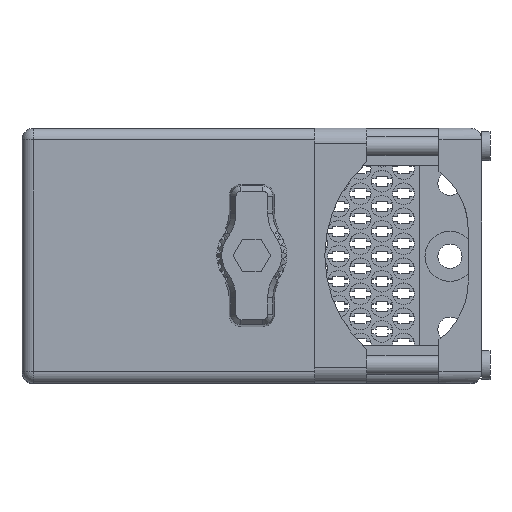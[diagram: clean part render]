
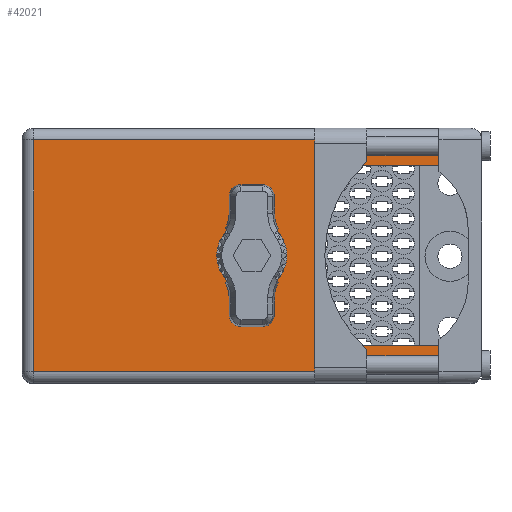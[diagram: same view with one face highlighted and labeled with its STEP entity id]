
A CAD part, top view. The second image highlights one B-rep face of the part: STEP entity #42021.
In plain terms, the highlighted face is planar.
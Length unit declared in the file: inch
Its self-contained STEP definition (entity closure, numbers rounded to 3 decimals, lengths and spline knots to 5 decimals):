
#489 = CARTESIAN_POINT ( 'NONE',  ( 0.4075, 1.93, -0.54 ) ) ;
#1414 = ORIENTED_EDGE ( 'NONE', *, *, #18481, .F. ) ;
#3510 = LINE ( 'NONE', #55622, #70464 ) ;
#4238 = FACE_OUTER_BOUND ( 'NONE', #34804, .T. ) ;
#4299 = VERTEX_POINT ( 'NONE', #4858 ) ;
#4858 = CARTESIAN_POINT ( 'NONE',  ( 1.1215, 1.93, -0.54 ) ) ;
#5364 = DIRECTION ( 'NONE',  ( 0., 0., 1. ) ) ;
#6829 = DIRECTION ( 'NONE',  ( 1., 0., 0. ) ) ;
#6981 = CARTESIAN_POINT ( 'NONE',  ( 1.1215, 1.93, -0.765 ) ) ;
#7824 = DIRECTION ( 'NONE',  ( 0., 1., 0. ) ) ;
#9221 = LINE ( 'NONE', #51453, #51146 ) ;
#11027 = ORIENTED_EDGE ( 'NONE', *, *, #24047, .F. ) ;
#11509 = ORIENTED_EDGE ( 'NONE', *, *, #74046, .F. ) ;
#11756 = DIRECTION ( 'NONE',  ( 0., 0., 1. ) ) ;
#12356 = ORIENTED_EDGE ( 'NONE', *, *, #43190, .T. ) ;
#15482 = CARTESIAN_POINT ( 'NONE',  ( 1.1215, 1.93, -0.695 ) ) ;
#15818 = VERTEX_POINT ( 'NONE', #64501 ) ;
#15840 = DIRECTION ( 'NONE',  ( 0., 0., 1. ) ) ;
#16463 = CARTESIAN_POINT ( 'NONE',  ( -1.3075, 1.93, -0.765 ) ) ;
#17051 = VECTOR ( 'NONE', #6829, 39.37008 ) ;
#18307 = DIRECTION ( 'NONE',  ( -1., 0., 0. ) ) ;
#18397 = CARTESIAN_POINT ( 'NONE',  ( 1.1215, 1.93, -0.765 ) ) ;
#18452 = VERTEX_POINT ( 'NONE', #19703 ) ;
#18481 = EDGE_CURVE ( 'NONE', #60884, #58365, #86616, .T. ) ;
#19607 = VERTEX_POINT ( 'NONE', #54149 ) ;
#19703 = CARTESIAN_POINT ( 'NONE',  ( 1.1215, 1.93, 0.54 ) ) ;
#24047 = EDGE_CURVE ( 'NONE', #58365, #60884, #51631, .T. ) ;
#24074 = VERTEX_POINT ( 'NONE', #76144 ) ;
#25149 = DIRECTION ( 'NONE',  ( 1., 0., 0. ) ) ;
#25889 = VERTEX_POINT ( 'NONE', #37792 ) ;
#26340 = CARTESIAN_POINT ( 'NONE',  ( 1.1215, 1.93, 0.54 ) ) ;
#26749 = VERTEX_POINT ( 'NONE', #50047 ) ;
#28099 = VERTEX_POINT ( 'NONE', #15482 ) ;
#31856 = EDGE_CURVE ( 'NONE', #25889, #26749, #66881, .T. ) ;
#32583 = ORIENTED_EDGE ( 'NONE', *, *, #47386, .T. ) ;
#33002 = LINE ( 'NONE', #18397, #38907 ) ;
#33477 = DIRECTION ( 'NONE',  ( -1., 0., 0. ) ) ;
#34354 = EDGE_CURVE ( 'NONE', #19607, #15818, #55673, .T. ) ;
#34804 = EDGE_LOOP ( 'NONE', ( #63378, #39633, #59728, #93427, #61352, #12356, #11509, #32583 ) ) ;
#37792 = CARTESIAN_POINT ( 'NONE',  ( 0.4075, 1.93, 0.54 ) ) ;
#38254 = CARTESIAN_POINT ( 'NONE',  ( 0., 1.93, 0. ) ) ;
#38815 = VECTOR ( 'NONE', #61947, 39.37008 ) ;
#38907 = VECTOR ( 'NONE', #11756, 39.37008 ) ;
#39633 = ORIENTED_EDGE ( 'NONE', *, *, #98437, .T. ) ;
#39798 = CARTESIAN_POINT ( 'NONE',  ( 0., 1.93, 0.17 ) ) ;
#40092 = AXIS2_PLACEMENT_3D ( 'NONE', #38254, #7824, #15840 ) ;
#42021 = ADVANCED_FACE ( 'NONE', ( #4238, #61637 ), #95406, .T. ) ;
#43190 = EDGE_CURVE ( 'NONE', #26749, #4299, #98501, .T. ) ;
#43706 = CARTESIAN_POINT ( 'NONE',  ( 0., 1.93, -0.17 ) ) ;
#47386 = EDGE_CURVE ( 'NONE', #28099, #19607, #9221, .T. ) ;
#49927 = DIRECTION ( 'NONE',  ( 0., 1., 0. ) ) ;
#50047 = CARTESIAN_POINT ( 'NONE',  ( 0.4075, 1.93, -0.54 ) ) ;
#51146 = VECTOR ( 'NONE', #59412, 39.37008 ) ;
#51198 = DIRECTION ( 'NONE',  ( 0., 1., 0. ) ) ;
#51453 = CARTESIAN_POINT ( 'NONE',  ( -1.3775, 1.93, -0.695 ) ) ;
#51631 = CIRCLE ( 'NONE', #40092, 0.17 ) ;
#52237 = EDGE_CURVE ( 'NONE', #18452, #25889, #86073, .T. ) ;
#53761 = LINE ( 'NONE', #6981, #69246 ) ;
#53992 = DIRECTION ( 'NONE',  ( 0., 0., -1. ) ) ;
#54149 = CARTESIAN_POINT ( 'NONE',  ( -1.3075, 1.93, -0.695 ) ) ;
#54759 = EDGE_LOOP ( 'NONE', ( #1414, #11027 ) ) ;
#55622 = CARTESIAN_POINT ( 'NONE',  ( 1.1215, 1.93, 0.695 ) ) ;
#55673 = LINE ( 'NONE', #16463, #38815 ) ;
#58365 = VERTEX_POINT ( 'NONE', #43706 ) ;
#59147 = DIRECTION ( 'NONE',  ( 0., 0., 1. ) ) ;
#59412 = DIRECTION ( 'NONE',  ( -1., 0., 0. ) ) ;
#59728 = ORIENTED_EDGE ( 'NONE', *, *, #72069, .F. ) ;
#60884 = VERTEX_POINT ( 'NONE', #39798 ) ;
#60897 = VECTOR ( 'NONE', #53992, 39.37008 ) ;
#61343 = AXIS2_PLACEMENT_3D ( 'NONE', #87983, #51198, #5364 ) ;
#61352 = ORIENTED_EDGE ( 'NONE', *, *, #31856, .T. ) ;
#61637 = FACE_BOUND ( 'NONE', #54759, .T. ) ;
#61947 = DIRECTION ( 'NONE',  ( 0., 0., 1. ) ) ;
#63378 = ORIENTED_EDGE ( 'NONE', *, *, #34354, .T. ) ;
#64501 = CARTESIAN_POINT ( 'NONE',  ( -1.3075, 1.93, 0.695 ) ) ;
#66881 = LINE ( 'NONE', #489, #60897 ) ;
#69246 = VECTOR ( 'NONE', #59147, 39.37008 ) ;
#70464 = VECTOR ( 'NONE', #25149, 39.37008 ) ;
#72069 = EDGE_CURVE ( 'NONE', #18452, #24074, #53761, .T. ) ;
#74046 = EDGE_CURVE ( 'NONE', #28099, #4299, #33002, .T. ) ;
#76144 = CARTESIAN_POINT ( 'NONE',  ( 1.1215, 1.93, 0.695 ) ) ;
#81296 = VECTOR ( 'NONE', #18307, 39.37008 ) ;
#86073 = LINE ( 'NONE', #26340, #81296 ) ;
#86616 = CIRCLE ( 'NONE', #61343, 0.17 ) ;
#87983 = CARTESIAN_POINT ( 'NONE',  ( 0., 1.93, 0. ) ) ;
#93427 = ORIENTED_EDGE ( 'NONE', *, *, #52237, .T. ) ;
#95063 = CARTESIAN_POINT ( 'NONE',  ( -1.3775, 1.93, -0.765 ) ) ;
#95406 = PLANE ( 'NONE',  #97130 ) ;
#97130 = AXIS2_PLACEMENT_3D ( 'NONE', #95063, #49927, #33477 ) ;
#97831 = CARTESIAN_POINT ( 'NONE',  ( 1.1215, 1.93, -0.54 ) ) ;
#98437 = EDGE_CURVE ( 'NONE', #15818, #24074, #3510, .T. ) ;
#98501 = LINE ( 'NONE', #97831, #17051 ) ;
